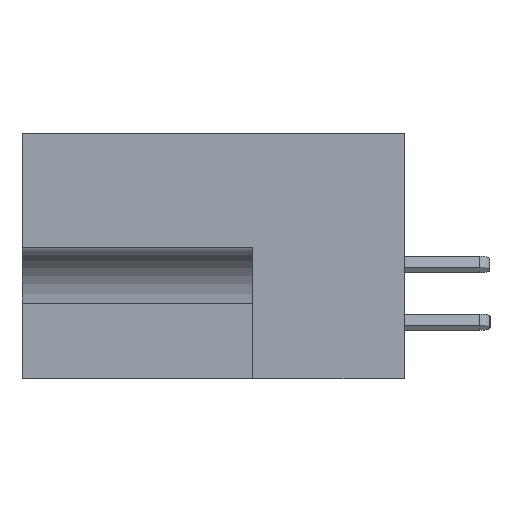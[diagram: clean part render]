
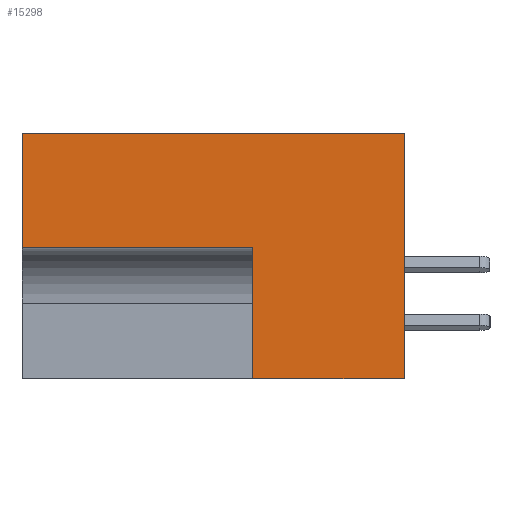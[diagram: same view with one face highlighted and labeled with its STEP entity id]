
A CAD part, left-side view. The second image highlights one B-rep face of the part: STEP entity #15298.
In plain terms, the highlighted planar face has unit normal (-1, 0, 0).
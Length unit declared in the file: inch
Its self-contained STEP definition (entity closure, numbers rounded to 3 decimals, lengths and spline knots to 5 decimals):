
#54 = VERTEX_POINT ( 'NONE', #2571 ) ;
#93 = LINE ( 'NONE', #22436, #6561 ) ;
#1721 = EDGE_CURVE ( 'NONE', #8954, #54, #93, .T. ) ;
#2383 = VECTOR ( 'NONE', #21435, 39.37008 ) ;
#2571 = CARTESIAN_POINT ( 'NONE',  ( 0., 0., 0. ) ) ;
#2763 = DIRECTION ( 'NONE',  ( 0., -1., 0. ) ) ;
#3067 = LINE ( 'NONE', #26072, #6947 ) ;
#3394 = EDGE_CURVE ( 'NONE', #7442, #8954, #7444, .T. ) ;
#4552 = EDGE_LOOP ( 'NONE', ( #18618, #11287, #22816, #25633, #5855, #6994 ) ) ;
#5855 = ORIENTED_EDGE ( 'NONE', *, *, #1721, .T. ) ;
#6494 = CARTESIAN_POINT ( 'NONE',  ( 0., 0.453, 0. ) ) ;
#6544 = CARTESIAN_POINT ( 'NONE',  ( 0., 0.453, 0. ) ) ;
#6561 = VECTOR ( 'NONE', #24620, 39.37008 ) ;
#6635 = LINE ( 'NONE', #15035, #11522 ) ;
#6947 = VECTOR ( 'NONE', #16219, 39.37008 ) ;
#6994 = ORIENTED_EDGE ( 'NONE', *, *, #21024, .F. ) ;
#7442 = VERTEX_POINT ( 'NONE', #18090 ) ;
#7444 = LINE ( 'NONE', #18307, #13306 ) ;
#7762 = AXIS2_PLACEMENT_3D ( 'NONE', #6544, #16855, #25404 ) ;
#8379 = CARTESIAN_POINT ( 'NONE',  ( 0., 0.828, 0. ) ) ;
#8954 = VERTEX_POINT ( 'NONE', #15633 ) ;
#11057 = FACE_OUTER_BOUND ( 'NONE', #4552, .T. ) ;
#11287 = ORIENTED_EDGE ( 'NONE', *, *, #21445, .F. ) ;
#11522 = VECTOR ( 'NONE', #22623, 39.37008 ) ;
#13005 = EDGE_CURVE ( 'NONE', #7442, #17040, #6635, .T. ) ;
#13193 = CARTESIAN_POINT ( 'NONE',  ( 0., 0.328, -0.248 ) ) ;
#13306 = VECTOR ( 'NONE', #22685, 39.37008 ) ;
#13794 = LINE ( 'NONE', #6494, #24228 ) ;
#13916 = VERTEX_POINT ( 'NONE', #20438 ) ;
#15035 = CARTESIAN_POINT ( 'NONE',  ( 0., 0.328, -0.531 ) ) ;
#15298 = ADVANCED_FACE ( 'NONE', ( #11057 ), #18952, .F. ) ;
#15633 = CARTESIAN_POINT ( 'NONE',  ( 0., 0., -0.531 ) ) ;
#16219 = DIRECTION ( 'NONE',  ( 0., 0., 1. ) ) ;
#16855 = DIRECTION ( 'NONE',  ( 1., 0., 0. ) ) ;
#17040 = VERTEX_POINT ( 'NONE', #13193 ) ;
#18090 = CARTESIAN_POINT ( 'NONE',  ( 0., 0.328, -0.531 ) ) ;
#18307 = CARTESIAN_POINT ( 'NONE',  ( 0., 0.453, -0.531 ) ) ;
#18618 = ORIENTED_EDGE ( 'NONE', *, *, #23374, .F. ) ;
#18952 = PLANE ( 'NONE',  #7762 ) ;
#19257 = CARTESIAN_POINT ( 'NONE',  ( 0., 0.328, -0.248 ) ) ;
#20438 = CARTESIAN_POINT ( 'NONE',  ( 0., 0.828, -0.248 ) ) ;
#21024 = EDGE_CURVE ( 'NONE', #26239, #54, #13794, .T. ) ;
#21435 = DIRECTION ( 'NONE',  ( 0., 1., 0. ) ) ;
#21445 = EDGE_CURVE ( 'NONE', #17040, #13916, #26507, .T. ) ;
#22436 = CARTESIAN_POINT ( 'NONE',  ( 0., 0., 0. ) ) ;
#22623 = DIRECTION ( 'NONE',  ( 0., 0., 1. ) ) ;
#22685 = DIRECTION ( 'NONE',  ( 0., -1., 0. ) ) ;
#22816 = ORIENTED_EDGE ( 'NONE', *, *, #13005, .F. ) ;
#23374 = EDGE_CURVE ( 'NONE', #13916, #26239, #3067, .T. ) ;
#24228 = VECTOR ( 'NONE', #2763, 39.37008 ) ;
#24620 = DIRECTION ( 'NONE',  ( 0., 0., 1. ) ) ;
#25404 = DIRECTION ( 'NONE',  ( 0., 0., -1. ) ) ;
#25633 = ORIENTED_EDGE ( 'NONE', *, *, #3394, .T. ) ;
#26072 = CARTESIAN_POINT ( 'NONE',  ( 0., 0.828, 0. ) ) ;
#26239 = VERTEX_POINT ( 'NONE', #8379 ) ;
#26507 = LINE ( 'NONE', #19257, #2383 ) ;
